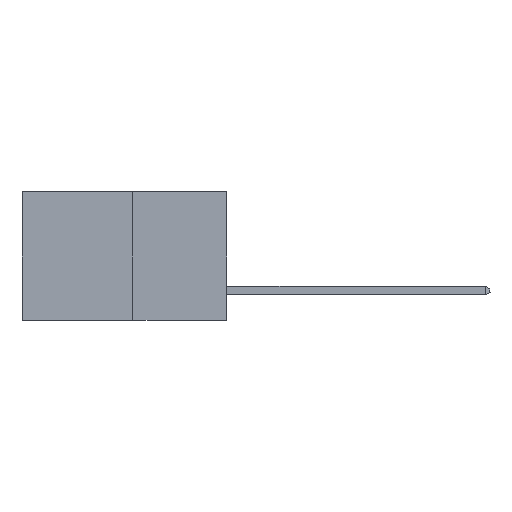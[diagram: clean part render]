
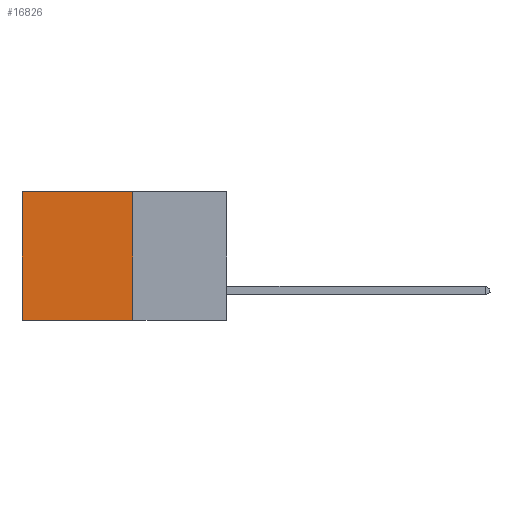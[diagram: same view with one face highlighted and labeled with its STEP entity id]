
A CAD part, left-side view. The second image highlights one B-rep face of the part: STEP entity #16826.
In plain terms, the highlighted planar face has unit normal (-1, 0, 0).
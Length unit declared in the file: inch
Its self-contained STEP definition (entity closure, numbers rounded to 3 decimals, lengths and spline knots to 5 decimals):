
#59 = CARTESIAN_POINT ( 'NONE',  ( 0.277, 0.27, -0.37 ) ) ;
#284 = ORIENTED_EDGE ( 'NONE', *, *, #6627, .F. ) ;
#389 = DIRECTION ( 'NONE',  ( 0., 1., 0. ) ) ;
#627 = AXIS2_PLACEMENT_3D ( 'NONE', #59, #2560, #19761 ) ;
#1589 = VECTOR ( 'NONE', #1815, 39.37008 ) ;
#1815 = DIRECTION ( 'NONE',  ( 0., 0., -1. ) ) ;
#2560 = DIRECTION ( 'NONE',  ( 1., 0., 0. ) ) ;
#3584 = CARTESIAN_POINT ( 'NONE',  ( 0.277, 0.27, 0. ) ) ;
#4215 = CARTESIAN_POINT ( 'NONE',  ( 0.277, 0.59, -0.37 ) ) ;
#5175 = VERTEX_POINT ( 'NONE', #5438 ) ;
#5438 = CARTESIAN_POINT ( 'NONE',  ( 0.277, 0.27, -0.37 ) ) ;
#6627 = EDGE_CURVE ( 'NONE', #14964, #5175, #16401, .T. ) ;
#7013 = LINE ( 'NONE', #3584, #19339 ) ;
#8093 = LINE ( 'NONE', #4215, #1589 ) ;
#12675 = FACE_OUTER_BOUND ( 'NONE', #24108, .T. ) ;
#12898 = EDGE_CURVE ( 'NONE', #25482, #15318, #8093, .T. ) ;
#13177 = EDGE_CURVE ( 'NONE', #5175, #15318, #13463, .T. ) ;
#13319 = DIRECTION ( 'NONE',  ( 0., 1., 0. ) ) ;
#13463 = LINE ( 'NONE', #17470, #25004 ) ;
#14964 = VERTEX_POINT ( 'NONE', #17353 ) ;
#15318 = VERTEX_POINT ( 'NONE', #28957 ) ;
#16401 = LINE ( 'NONE', #16606, #22221 ) ;
#16456 = DIRECTION ( 'NONE',  ( 0., 0., -1. ) ) ;
#16606 = CARTESIAN_POINT ( 'NONE',  ( 0.277, 0.27, -0.37 ) ) ;
#16826 = ADVANCED_FACE ( 'NONE', ( #12675 ), #17239, .F. ) ;
#17239 = PLANE ( 'NONE',  #627 ) ;
#17353 = CARTESIAN_POINT ( 'NONE',  ( 0.277, 0.27, 0. ) ) ;
#17470 = CARTESIAN_POINT ( 'NONE',  ( 0.277, 0.27, -0.37 ) ) ;
#17588 = ORIENTED_EDGE ( 'NONE', *, *, #13177, .F. ) ;
#19339 = VECTOR ( 'NONE', #13319, 39.37008 ) ;
#19761 = DIRECTION ( 'NONE',  ( 0., 0., -1. ) ) ;
#21484 = ORIENTED_EDGE ( 'NONE', *, *, #22038, .T. ) ;
#22038 = EDGE_CURVE ( 'NONE', #14964, #25482, #7013, .T. ) ;
#22221 = VECTOR ( 'NONE', #16456, 39.37008 ) ;
#22612 = ORIENTED_EDGE ( 'NONE', *, *, #12898, .T. ) ;
#23347 = CARTESIAN_POINT ( 'NONE',  ( 0.277, 0.59, 0. ) ) ;
#24108 = EDGE_LOOP ( 'NONE', ( #22612, #17588, #284, #21484 ) ) ;
#25004 = VECTOR ( 'NONE', #389, 39.37008 ) ;
#25482 = VERTEX_POINT ( 'NONE', #23347 ) ;
#28957 = CARTESIAN_POINT ( 'NONE',  ( 0.277, 0.59, -0.37 ) ) ;
